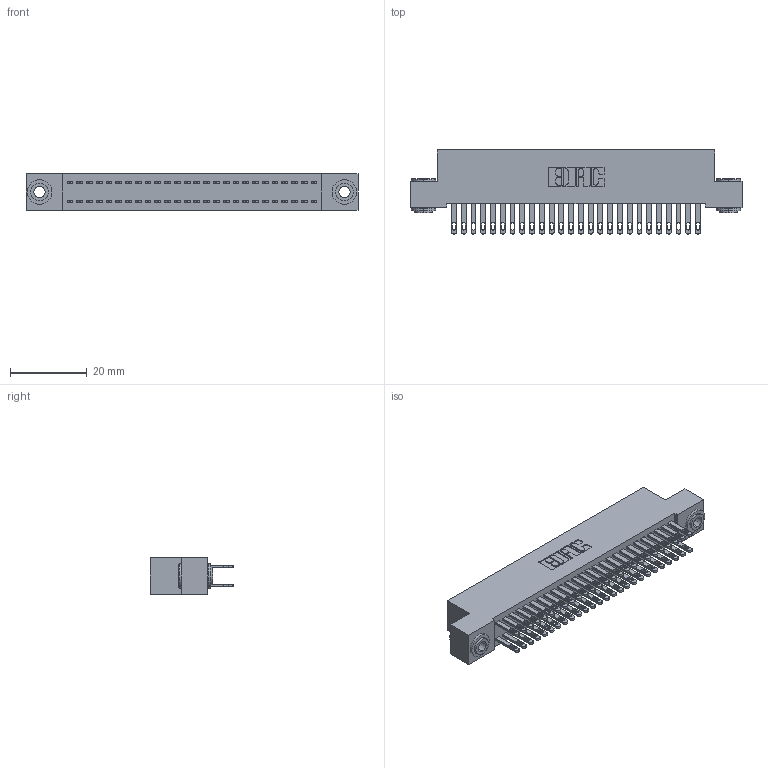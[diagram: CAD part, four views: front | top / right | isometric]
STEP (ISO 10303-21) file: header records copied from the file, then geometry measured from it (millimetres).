
FILE_DESCRIPTION (( 'STEP AP203' ), '1' );
FILE_NAME ('892-052-500-203.STEP', '2020-09-21T18:08:08', ( '' ), ( '' ), 'SwSTEP 2.0', 'SolidWorks 2020', '' );
FILE_SCHEMA (( 'CONFIG_CONTROL_DESIGN' ));
Length unit declared in the file: inch
Products named in the file (4): 342-250-002_345-250-002-102; 892-052-500-203; 842 Part_.156 TH; 345-292-001_345-293-100
Assembly tree (55 placements, depth 2):
  892-052-500-203
    842 Part_.156 TH
    345-292-001_345-293-100  x52
    342-250-002_345-250-002-102  x2
Bounding box: 86.36 x 21.85 x 9.4 mm (x, y, z)
Volume: 7865.4 mm3; surface area: 13120.6 mm2
Topology: 55 solids, 55 shells, 2644 faces, 8019 edges, 5342 vertices
Faces by surface type: plane 1636, cylinder 1000, cone 8
Entity records: 19244 total; most frequent: CARTESIAN_POINT 3181, ORIENTED_EDGE 3110, DIRECTION 2781, EDGE_CURVE 1555, VECTOR 1399, LINE 1399, VERTEX_POINT 1034, AXIS2_PLACEMENT_3D 691
